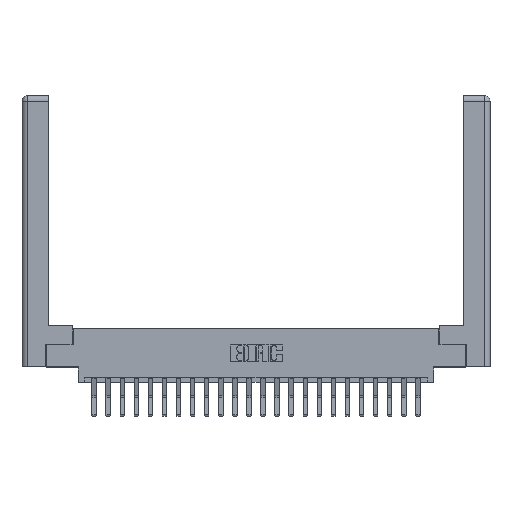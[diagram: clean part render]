
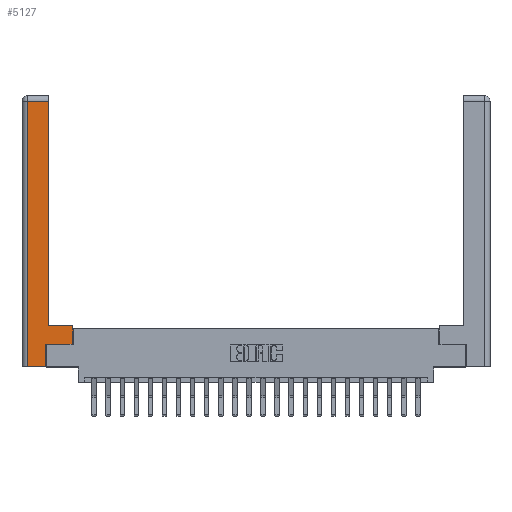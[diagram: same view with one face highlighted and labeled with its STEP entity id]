
A CAD part, top view. The second image highlights one B-rep face of the part: STEP entity #5127.
In plain terms, the highlighted planar face has unit normal (0, 0, 1).
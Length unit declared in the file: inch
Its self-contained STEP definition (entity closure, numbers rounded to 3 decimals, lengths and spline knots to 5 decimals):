
#3 = LINE ( 'NONE', #4850, #17570 ) ;
#81 = CARTESIAN_POINT ( 'NONE',  ( 0.565, 0.245, 0. ) ) ;
#169 = DIRECTION ( 'NONE',  ( -1., 0., 0. ) ) ;
#1022 = VECTOR ( 'NONE', #21543, 39.37008 ) ;
#3020 = EDGE_CURVE ( 'NONE', #4993, #4804, #3475, .T. ) ;
#3053 = VERTEX_POINT ( 'NONE', #8801 ) ;
#3125 = DIRECTION ( 'NONE',  ( 0., 1., 0. ) ) ;
#3475 = LINE ( 'NONE', #5022, #15860 ) ;
#3537 = CARTESIAN_POINT ( 'NONE',  ( 0.0615, 2.94, 0. ) ) ;
#4216 = DIRECTION ( 'NONE',  ( -1., 0., 0. ) ) ;
#4221 = LINE ( 'NONE', #5257, #7094 ) ;
#4608 = VECTOR ( 'NONE', #169, 39.37008 ) ;
#4804 = VERTEX_POINT ( 'NONE', #7568 ) ;
#4850 = CARTESIAN_POINT ( 'NONE',  ( 0.295, 0.45, 0. ) ) ;
#4853 = LINE ( 'NONE', #22632, #9740 ) ;
#4993 = VERTEX_POINT ( 'NONE', #18049 ) ;
#5022 = CARTESIAN_POINT ( 'NONE',  ( 0.265, 0., 0. ) ) ;
#5127 = ADVANCED_FACE ( 'NONE', ( #21779 ), #13381, .F. ) ;
#5244 = CARTESIAN_POINT ( 'NONE',  ( 0.0615, 0., 0. ) ) ;
#5257 = CARTESIAN_POINT ( 'NONE',  ( 0.565, 0.245, 0. ) ) ;
#5692 = ORIENTED_EDGE ( 'NONE', *, *, #11924, .T. ) ;
#5882 = ORIENTED_EDGE ( 'NONE', *, *, #12552, .T. ) ;
#5978 = EDGE_CURVE ( 'NONE', #13808, #7079, #4221, .T. ) ;
#6481 = LINE ( 'NONE', #16140, #1022 ) ;
#7079 = VERTEX_POINT ( 'NONE', #81 ) ;
#7094 = VECTOR ( 'NONE', #16233, 39.37008 ) ;
#7236 = VECTOR ( 'NONE', #14658, 39.37008 ) ;
#7568 = CARTESIAN_POINT ( 'NONE',  ( 0.265, 0., 0. ) ) ;
#7721 = ORIENTED_EDGE ( 'NONE', *, *, #5978, .T. ) ;
#7764 = CARTESIAN_POINT ( 'NONE',  ( 0.295, 2.94, 0. ) ) ;
#8801 = CARTESIAN_POINT ( 'NONE',  ( 0.565, 0.45, 0. ) ) ;
#9079 = EDGE_CURVE ( 'NONE', #20501, #21429, #6481, .T. ) ;
#9717 = LINE ( 'NONE', #15846, #17524 ) ;
#9740 = VECTOR ( 'NONE', #15021, 39.37008 ) ;
#11221 = LINE ( 'NONE', #3537, #4608 ) ;
#11924 = EDGE_CURVE ( 'NONE', #13793, #4993, #22479, .T. ) ;
#12351 = DIRECTION ( 'NONE',  ( 1., 0., 0. ) ) ;
#12552 = EDGE_CURVE ( 'NONE', #21429, #13793, #11221, .T. ) ;
#13222 = EDGE_CURVE ( 'NONE', #7079, #3053, #4853, .T. ) ;
#13381 = PLANE ( 'NONE',  #15340 ) ;
#13459 = CARTESIAN_POINT ( 'NONE',  ( 0., 0., 0. ) ) ;
#13793 = VERTEX_POINT ( 'NONE', #19948 ) ;
#13808 = VERTEX_POINT ( 'NONE', #21783 ) ;
#14658 = DIRECTION ( 'NONE',  ( 0., -1., 0. ) ) ;
#14659 = ORIENTED_EDGE ( 'NONE', *, *, #9079, .T. ) ;
#15021 = DIRECTION ( 'NONE',  ( 0., 1., 0. ) ) ;
#15077 = DIRECTION ( 'NONE',  ( 0., 0., -1. ) ) ;
#15340 = AXIS2_PLACEMENT_3D ( 'NONE', #13459, #15077, #4216 ) ;
#15846 = CARTESIAN_POINT ( 'NONE',  ( 0.265, 0.245, 0. ) ) ;
#15860 = VECTOR ( 'NONE', #12351, 39.37008 ) ;
#16140 = CARTESIAN_POINT ( 'NONE',  ( 0.295, 3., 0. ) ) ;
#16233 = DIRECTION ( 'NONE',  ( 1., 0., 0. ) ) ;
#17030 = EDGE_CURVE ( 'NONE', #4804, #13808, #9717, .T. ) ;
#17524 = VECTOR ( 'NONE', #3125, 39.37008 ) ;
#17570 = VECTOR ( 'NONE', #23102, 39.37008 ) ;
#18049 = CARTESIAN_POINT ( 'NONE',  ( 0.0615, 0., 0. ) ) ;
#19196 = ORIENTED_EDGE ( 'NONE', *, *, #17030, .T. ) ;
#19843 = ORIENTED_EDGE ( 'NONE', *, *, #23648, .T. ) ;
#19948 = CARTESIAN_POINT ( 'NONE',  ( 0.0615, 2.94, 0. ) ) ;
#20501 = VERTEX_POINT ( 'NONE', #23676 ) ;
#21252 = EDGE_LOOP ( 'NONE', ( #14659, #5882, #5692, #21909, #19196, #7721, #23088, #19843 ) ) ;
#21429 = VERTEX_POINT ( 'NONE', #7764 ) ;
#21543 = DIRECTION ( 'NONE',  ( 0., 1., 0. ) ) ;
#21779 = FACE_OUTER_BOUND ( 'NONE', #21252, .T. ) ;
#21783 = CARTESIAN_POINT ( 'NONE',  ( 0.265, 0.245, 0. ) ) ;
#21909 = ORIENTED_EDGE ( 'NONE', *, *, #3020, .T. ) ;
#22479 = LINE ( 'NONE', #5244, #7236 ) ;
#22632 = CARTESIAN_POINT ( 'NONE',  ( 0.565, 0.45, 0. ) ) ;
#23088 = ORIENTED_EDGE ( 'NONE', *, *, #13222, .T. ) ;
#23102 = DIRECTION ( 'NONE',  ( -1., 0., 0. ) ) ;
#23648 = EDGE_CURVE ( 'NONE', #3053, #20501, #3, .T. ) ;
#23676 = CARTESIAN_POINT ( 'NONE',  ( 0.295, 0.45, 0. ) ) ;
